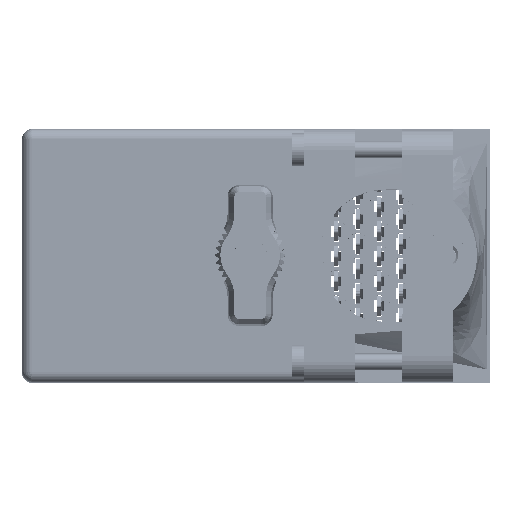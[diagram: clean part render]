
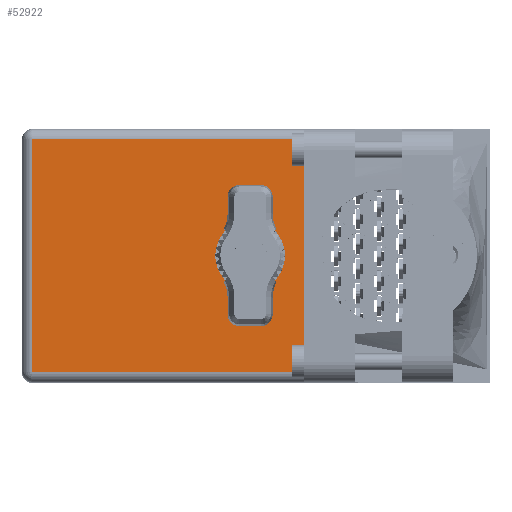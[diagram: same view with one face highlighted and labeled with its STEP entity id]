
A CAD part, top view. The second image highlights one B-rep face of the part: STEP entity #52922.
In plain terms, the highlighted face is planar.
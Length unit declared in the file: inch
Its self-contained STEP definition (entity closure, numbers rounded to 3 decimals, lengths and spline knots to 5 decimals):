
#156 = VERTEX_POINT ( 'NONE', #49199 ) ;
#903 = DIRECTION ( 'NONE',  ( 0., 0., 1. ) ) ;
#940 = DIRECTION ( 'NONE',  ( 1., 0., 0. ) ) ;
#2399 = FACE_OUTER_BOUND ( 'NONE', #21656, .T. ) ;
#3271 = ORIENTED_EDGE ( 'NONE', *, *, #83075, .T. ) ;
#4338 = CARTESIAN_POINT ( 'NONE',  ( 0.062, 2.03, -0.062 ) ) ;
#4985 = VERTEX_POINT ( 'NONE', #114383 ) ;
#8220 = VERTEX_POINT ( 'NONE', #34851 ) ;
#9673 = LINE ( 'NONE', #57600, #84506 ) ;
#12855 = CIRCLE ( 'NONE', #85761, 0.1015 ) ;
#17280 = AXIS2_PLACEMENT_3D ( 'NONE', #115952, #80231, #25935 ) ;
#18356 = CIRCLE ( 'NONE', #17280, 0.1015 ) ;
#20625 = DIRECTION ( 'NONE',  ( 0., 0., 1. ) ) ;
#21160 = ORIENTED_EDGE ( 'NONE', *, *, #82336, .F. ) ;
#21656 = EDGE_LOOP ( 'NONE', ( #90265, #97673, #105215, #3271 ) ) ;
#25935 = DIRECTION ( 'NONE',  ( 0., 0., 1. ) ) ;
#28298 = FACE_BOUND ( 'NONE', #78959, .T. ) ;
#29558 = EDGE_CURVE ( 'NONE', #66393, #36241, #59866, .T. ) ;
#34851 = CARTESIAN_POINT ( 'NONE',  ( 1.705, 2.03, -0.062 ) ) ;
#34897 = DIRECTION ( 'NONE',  ( 0., 1., 0. ) ) ;
#36241 = VERTEX_POINT ( 'NONE', #4338 ) ;
#36494 = AXIS2_PLACEMENT_3D ( 'NONE', #69438, #97985, #79868 ) ;
#37447 = CARTESIAN_POINT ( 'NONE',  ( 0.062, 2.03, -1.53 ) ) ;
#44064 = VECTOR ( 'NONE', #903, 39.37008 ) ;
#49199 = CARTESIAN_POINT ( 'NONE',  ( 1.3775, 2.03, -0.8665 ) ) ;
#50337 = CARTESIAN_POINT ( 'NONE',  ( 0.062, 2.03, -1.468 ) ) ;
#52104 = PLANE ( 'NONE',  #36494 ) ;
#52922 = ADVANCED_FACE ( 'NONE', ( #2399, #28298 ), #52104, .T. ) ;
#53210 = EDGE_CURVE ( 'NONE', #36241, #8220, #108777, .T. ) ;
#53349 = DIRECTION ( 'NONE',  ( 0., 0., 1. ) ) ;
#55936 = CARTESIAN_POINT ( 'NONE',  ( 1.705, 2.03, -0.062 ) ) ;
#57600 = CARTESIAN_POINT ( 'NONE',  ( 1.705, 2.03, -1.53 ) ) ;
#57664 = CARTESIAN_POINT ( 'NONE',  ( 1.705, 2.03, -1.468 ) ) ;
#59866 = LINE ( 'NONE', #37447, #44064 ) ;
#62531 = DIRECTION ( 'NONE',  ( -1., 0., 0. ) ) ;
#66393 = VERTEX_POINT ( 'NONE', #50337 ) ;
#69438 = CARTESIAN_POINT ( 'NONE',  ( 0., 2.03, -1.53 ) ) ;
#78959 = EDGE_LOOP ( 'NONE', ( #21160, #92681 ) ) ;
#79868 = DIRECTION ( 'NONE',  ( 0., 0., 1. ) ) ;
#80231 = DIRECTION ( 'NONE',  ( 0., 1., 0. ) ) ;
#82336 = EDGE_CURVE ( 'NONE', #4985, #156, #12855, .T. ) ;
#83075 = EDGE_CURVE ( 'NONE', #90613, #66393, #83090, .T. ) ;
#83090 = LINE ( 'NONE', #107508, #110379 ) ;
#83187 = EDGE_CURVE ( 'NONE', #156, #4985, #18356, .T. ) ;
#84506 = VECTOR ( 'NONE', #20625, 39.37008 ) ;
#85761 = AXIS2_PLACEMENT_3D ( 'NONE', #98825, #34897, #53349 ) ;
#90265 = ORIENTED_EDGE ( 'NONE', *, *, #29558, .T. ) ;
#90613 = VERTEX_POINT ( 'NONE', #57664 ) ;
#92681 = ORIENTED_EDGE ( 'NONE', *, *, #83187, .F. ) ;
#94424 = VECTOR ( 'NONE', #940, 39.37008 ) ;
#97673 = ORIENTED_EDGE ( 'NONE', *, *, #53210, .T. ) ;
#97985 = DIRECTION ( 'NONE',  ( 0., 1., 0. ) ) ;
#98825 = CARTESIAN_POINT ( 'NONE',  ( 1.3775, 2.03, -0.765 ) ) ;
#105215 = ORIENTED_EDGE ( 'NONE', *, *, #114491, .F. ) ;
#107508 = CARTESIAN_POINT ( 'NONE',  ( 0., 2.03, -1.468 ) ) ;
#108777 = LINE ( 'NONE', #55936, #94424 ) ;
#110379 = VECTOR ( 'NONE', #62531, 39.37008 ) ;
#114383 = CARTESIAN_POINT ( 'NONE',  ( 1.3775, 2.03, -0.6635 ) ) ;
#114491 = EDGE_CURVE ( 'NONE', #90613, #8220, #9673, .T. ) ;
#115952 = CARTESIAN_POINT ( 'NONE',  ( 1.3775, 2.03, -0.765 ) ) ;
